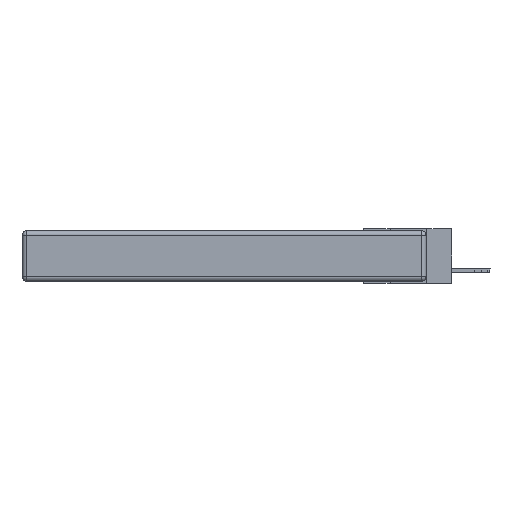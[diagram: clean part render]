
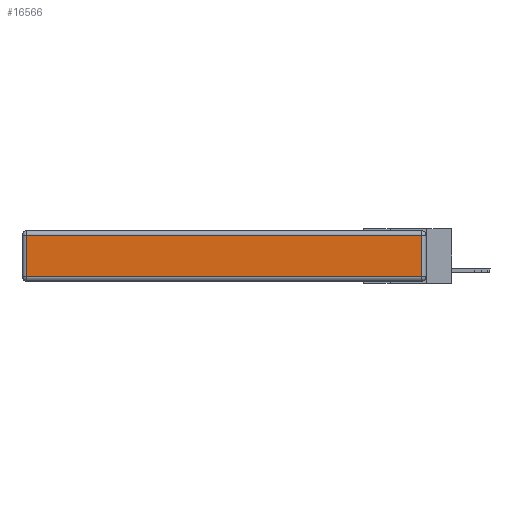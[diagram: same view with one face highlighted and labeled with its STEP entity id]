
A CAD part, left-side view. The second image highlights one B-rep face of the part: STEP entity #16566.
In plain terms, the highlighted planar face has unit normal (-1, 0, 0).
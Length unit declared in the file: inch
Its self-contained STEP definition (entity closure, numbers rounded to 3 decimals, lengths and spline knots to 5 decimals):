
#720 = ORIENTED_EDGE ( 'NONE', *, *, #16228, .T. ) ;
#855 = CARTESIAN_POINT ( 'NONE',  ( 0., 0.03, -0.343 ) ) ;
#1274 = CARTESIAN_POINT ( 'NONE',  ( 0., 0., -0.343 ) ) ;
#3309 = EDGE_CURVE ( 'NONE', #4593, #8177, #3716, .T. ) ;
#3716 = LINE ( 'NONE', #855, #13957 ) ;
#4002 = AXIS2_PLACEMENT_3D ( 'NONE', #1274, #19680, #18119 ) ;
#4593 = VERTEX_POINT ( 'NONE', #5012 ) ;
#5012 = CARTESIAN_POINT ( 'NONE',  ( 0., 0.03, -0.313 ) ) ;
#5644 = EDGE_CURVE ( 'NONE', #8177, #17712, #9117, .T. ) ;
#8177 = VERTEX_POINT ( 'NONE', #9039 ) ;
#8440 = CARTESIAN_POINT ( 'NONE',  ( 0., 2.72, -0.313 ) ) ;
#9039 = CARTESIAN_POINT ( 'NONE',  ( 0., 0.03, -0.03 ) ) ;
#9117 = LINE ( 'NONE', #22177, #10239 ) ;
#9557 = DIRECTION ( 'NONE',  ( 0., 1., 0. ) ) ;
#9640 = CARTESIAN_POINT ( 'NONE',  ( 0., 2.72, -0.343 ) ) ;
#9784 = ORIENTED_EDGE ( 'NONE', *, *, #11660, .T. ) ;
#10239 = VECTOR ( 'NONE', #9557, 39.37008 ) ;
#11218 = ORIENTED_EDGE ( 'NONE', *, *, #3309, .T. ) ;
#11300 = CARTESIAN_POINT ( 'NONE',  ( 0., 0., -0.313 ) ) ;
#11660 = EDGE_CURVE ( 'NONE', #17712, #13505, #18485, .T. ) ;
#11834 = DIRECTION ( 'NONE',  ( 0., -1., 0. ) ) ;
#13017 = DIRECTION ( 'NONE',  ( 0., 0., -1. ) ) ;
#13505 = VERTEX_POINT ( 'NONE', #8440 ) ;
#13957 = VECTOR ( 'NONE', #17166, 39.37008 ) ;
#14178 = CARTESIAN_POINT ( 'NONE',  ( 0., 2.72, -0.03 ) ) ;
#16228 = EDGE_CURVE ( 'NONE', #13505, #4593, #16711, .T. ) ;
#16566 = ADVANCED_FACE ( 'NONE', ( #21470 ), #19459, .T. ) ;
#16711 = LINE ( 'NONE', #11300, #22910 ) ;
#17166 = DIRECTION ( 'NONE',  ( 0., 0., 1. ) ) ;
#17524 = EDGE_LOOP ( 'NONE', ( #720, #11218, #21204, #9784 ) ) ;
#17712 = VERTEX_POINT ( 'NONE', #14178 ) ;
#18119 = DIRECTION ( 'NONE',  ( 0., 0., 1. ) ) ;
#18485 = LINE ( 'NONE', #9640, #19327 ) ;
#19327 = VECTOR ( 'NONE', #13017, 39.37008 ) ;
#19459 = PLANE ( 'NONE',  #4002 ) ;
#19680 = DIRECTION ( 'NONE',  ( -1., 0., 0. ) ) ;
#21204 = ORIENTED_EDGE ( 'NONE', *, *, #5644, .T. ) ;
#21470 = FACE_OUTER_BOUND ( 'NONE', #17524, .T. ) ;
#22177 = CARTESIAN_POINT ( 'NONE',  ( 0., 2.75, -0.03 ) ) ;
#22910 = VECTOR ( 'NONE', #11834, 39.37008 ) ;
